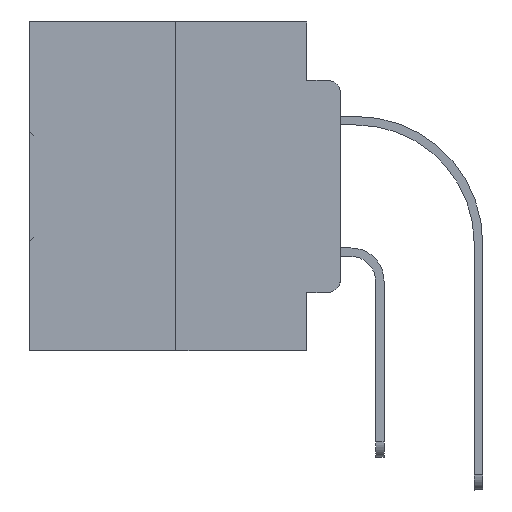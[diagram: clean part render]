
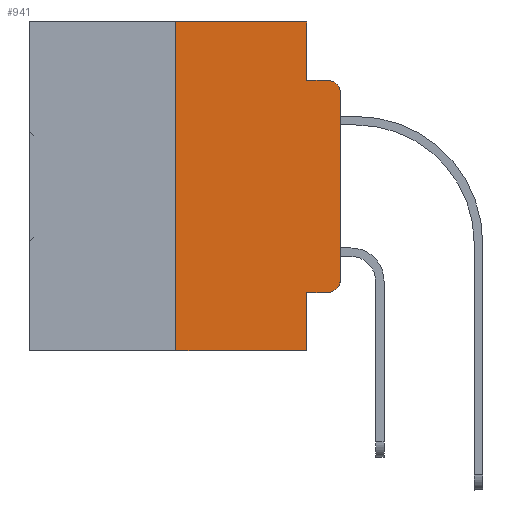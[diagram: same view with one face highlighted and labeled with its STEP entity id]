
A CAD part, left-side view. The second image highlights one B-rep face of the part: STEP entity #941.
In plain terms, the highlighted planar face has unit normal (-1, 0, 0).
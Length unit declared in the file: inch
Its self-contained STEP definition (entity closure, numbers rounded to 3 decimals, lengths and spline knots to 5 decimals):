
#246 = DIRECTION ( 'NONE',  ( 1., 0., 0. ) ) ;
#370 = CARTESIAN_POINT ( 'NONE',  ( 0., 0.25, -0.5 ) ) ;
#468 = ORIENTED_EDGE ( 'NONE', *, *, #28243, .F. ) ;
#812 = CARTESIAN_POINT ( 'NONE',  ( 0., 0.473, -0.5 ) ) ;
#941 = ADVANCED_FACE ( 'NONE', ( #24489 ), #21654, .F. ) ;
#998 = VERTEX_POINT ( 'NONE', #21474 ) ;
#1059 = AXIS2_PLACEMENT_3D ( 'NONE', #32459, #246, #34950 ) ;
#1072 = LINE ( 'NONE', #25666, #21278 ) ;
#1453 = LINE ( 'NONE', #27990, #13744 ) ;
#1867 = CARTESIAN_POINT ( 'NONE',  ( 0., 0.473, 0. ) ) ;
#2258 = ORIENTED_EDGE ( 'NONE', *, *, #15749, .T. ) ;
#2370 = ORIENTED_EDGE ( 'NONE', *, *, #7194, .F. ) ;
#2448 = VECTOR ( 'NONE', #27530, 39.37008 ) ;
#2911 = DIRECTION ( 'NONE',  ( -1., 0., 0. ) ) ;
#2982 = VECTOR ( 'NONE', #9767, 39.37008 ) ;
#3089 = AXIS2_PLACEMENT_3D ( 'NONE', #3099, #2911, #32492 ) ;
#3099 = CARTESIAN_POINT ( 'NONE',  ( 0., 0.02, -0.3915 ) ) ;
#3497 = EDGE_CURVE ( 'NONE', #7602, #34326, #33428, .T. ) ;
#6491 = CIRCLE ( 'NONE', #3089, 0.02 ) ;
#6763 = EDGE_CURVE ( 'NONE', #22237, #29436, #1072, .T. ) ;
#6885 = VERTEX_POINT ( 'NONE', #7258 ) ;
#6887 = CIRCLE ( 'NONE', #23288, 0.02 ) ;
#7193 = DIRECTION ( 'NONE',  ( 0., -1., 0. ) ) ;
#7194 = EDGE_CURVE ( 'NONE', #25245, #22237, #16793, .T. ) ;
#7228 = DIRECTION ( 'NONE',  ( 0., 0., -1. ) ) ;
#7258 = CARTESIAN_POINT ( 'NONE',  ( 0., 0.25, 0. ) ) ;
#7602 = VERTEX_POINT ( 'NONE', #30717 ) ;
#7644 = CARTESIAN_POINT ( 'NONE',  ( 0., 0.051, -0.0885 ) ) ;
#9049 = DIRECTION ( 'NONE',  ( 0., 0., 1. ) ) ;
#9245 = CARTESIAN_POINT ( 'NONE',  ( 0., 0.25, 0. ) ) ;
#9252 = ORIENTED_EDGE ( 'NONE', *, *, #6763, .F. ) ;
#9767 = DIRECTION ( 'NONE',  ( 0., 0., 1. ) ) ;
#10410 = DIRECTION ( 'NONE',  ( 0., -1., 0. ) ) ;
#10629 = DIRECTION ( 'NONE',  ( -1., 0., 0. ) ) ;
#11360 = ORIENTED_EDGE ( 'NONE', *, *, #3497, .F. ) ;
#11798 = ORIENTED_EDGE ( 'NONE', *, *, #14201, .T. ) ;
#12302 = CARTESIAN_POINT ( 'NONE',  ( 0., 0.051, -0.5 ) ) ;
#13666 = VECTOR ( 'NONE', #10410, 39.37008 ) ;
#13744 = VECTOR ( 'NONE', #9049, 39.37008 ) ;
#14201 = EDGE_CURVE ( 'NONE', #21672, #32946, #1453, .T. ) ;
#14649 = CARTESIAN_POINT ( 'NONE',  ( 0., 0., -0.3915 ) ) ;
#14917 = LINE ( 'NONE', #9245, #2982 ) ;
#15749 = EDGE_CURVE ( 'NONE', #32946, #29436, #6887, .T. ) ;
#16076 = LINE ( 'NONE', #23864, #13666 ) ;
#16208 = VECTOR ( 'NONE', #17320, 39.37008 ) ;
#16555 = VECTOR ( 'NONE', #7193, 39.37008 ) ;
#16793 = LINE ( 'NONE', #22989, #16208 ) ;
#16862 = EDGE_CURVE ( 'NONE', #6885, #25245, #34612, .T. ) ;
#17239 = CARTESIAN_POINT ( 'NONE',  ( 0., 0.051, 0. ) ) ;
#17320 = DIRECTION ( 'NONE',  ( 0., 0., -1. ) ) ;
#17457 = ORIENTED_EDGE ( 'NONE', *, *, #29039, .T. ) ;
#18281 = EDGE_CURVE ( 'NONE', #998, #21672, #6491, .T. ) ;
#18776 = ORIENTED_EDGE ( 'NONE', *, *, #25951, .T. ) ;
#20121 = EDGE_LOOP ( 'NONE', ( #11798, #2258, #9252, #2370, #22100, #468, #17457, #11360, #18776, #33552 ) ) ;
#20899 = DIRECTION ( 'NONE',  ( 0., 0., -1. ) ) ;
#21278 = VECTOR ( 'NONE', #33118, 39.37008 ) ;
#21474 = CARTESIAN_POINT ( 'NONE',  ( 0., 0.02, -0.4115 ) ) ;
#21654 = PLANE ( 'NONE',  #1059 ) ;
#21672 = VERTEX_POINT ( 'NONE', #14649 ) ;
#22100 = ORIENTED_EDGE ( 'NONE', *, *, #16862, .F. ) ;
#22237 = VERTEX_POINT ( 'NONE', #7644 ) ;
#22989 = CARTESIAN_POINT ( 'NONE',  ( 0., 0.051, 0. ) ) ;
#23288 = AXIS2_PLACEMENT_3D ( 'NONE', #29207, #10629, #20899 ) ;
#23547 = CARTESIAN_POINT ( 'NONE',  ( 0., 0., -0.1085 ) ) ;
#23864 = CARTESIAN_POINT ( 'NONE',  ( 0., 0.051, -0.4115 ) ) ;
#24489 = FACE_OUTER_BOUND ( 'NONE', #20121, .T. ) ;
#25245 = VERTEX_POINT ( 'NONE', #17239 ) ;
#25419 = VERTEX_POINT ( 'NONE', #370 ) ;
#25666 = CARTESIAN_POINT ( 'NONE',  ( 0., 0.051, -0.0885 ) ) ;
#25951 = EDGE_CURVE ( 'NONE', #7602, #998, #16076, .T. ) ;
#26938 = VECTOR ( 'NONE', #7228, 39.37008 ) ;
#27530 = DIRECTION ( 'NONE',  ( 0., -1., 0. ) ) ;
#27990 = CARTESIAN_POINT ( 'NONE',  ( 0., 0., 0. ) ) ;
#28243 = EDGE_CURVE ( 'NONE', #25419, #6885, #14917, .T. ) ;
#29039 = EDGE_CURVE ( 'NONE', #25419, #34326, #30521, .T. ) ;
#29207 = CARTESIAN_POINT ( 'NONE',  ( 0., 0.02, -0.1085 ) ) ;
#29436 = VERTEX_POINT ( 'NONE', #32586 ) ;
#30521 = LINE ( 'NONE', #812, #2448 ) ;
#30717 = CARTESIAN_POINT ( 'NONE',  ( 0., 0.051, -0.4115 ) ) ;
#32459 = CARTESIAN_POINT ( 'NONE',  ( 0., 0.473, 0. ) ) ;
#32492 = DIRECTION ( 'NONE',  ( 0., 0., -1. ) ) ;
#32586 = CARTESIAN_POINT ( 'NONE',  ( 0., 0.02, -0.0885 ) ) ;
#32946 = VERTEX_POINT ( 'NONE', #23547 ) ;
#33118 = DIRECTION ( 'NONE',  ( 0., -1., 0. ) ) ;
#33428 = LINE ( 'NONE', #33789, #26938 ) ;
#33552 = ORIENTED_EDGE ( 'NONE', *, *, #18281, .T. ) ;
#33789 = CARTESIAN_POINT ( 'NONE',  ( 0., 0.051, 0. ) ) ;
#34326 = VERTEX_POINT ( 'NONE', #12302 ) ;
#34612 = LINE ( 'NONE', #1867, #16555 ) ;
#34950 = DIRECTION ( 'NONE',  ( 0., 0., -1. ) ) ;
